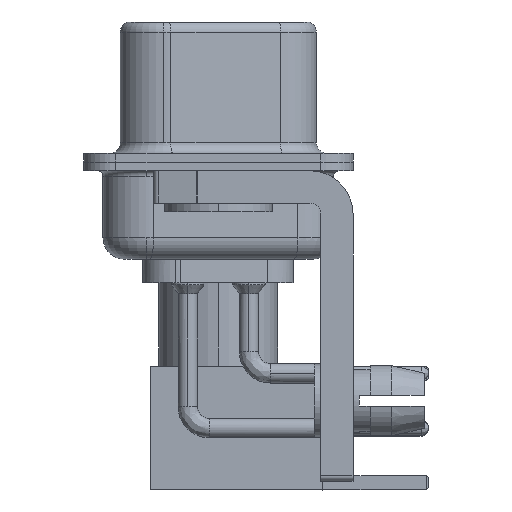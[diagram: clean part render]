
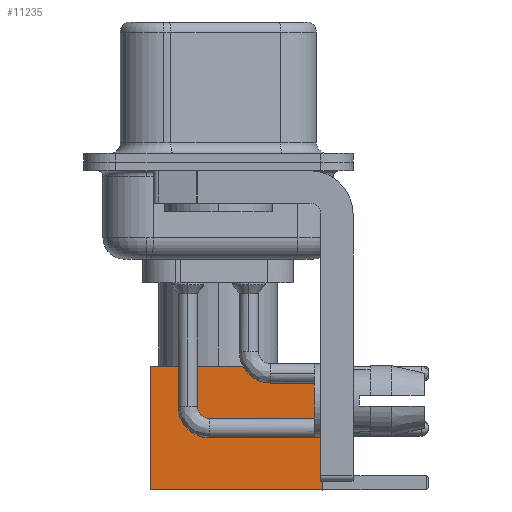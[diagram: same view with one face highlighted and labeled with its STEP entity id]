
A CAD part, left-side view. The second image highlights one B-rep face of the part: STEP entity #11235.
In plain terms, the highlighted face is planar.
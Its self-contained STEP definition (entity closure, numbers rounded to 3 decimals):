
#1261 = VERTEX_POINT ( 'NONE', #21179 ) ;
#3146 = VECTOR ( 'NONE', #19680, 1000. ) ;
#3464 = CARTESIAN_POINT ( 'NONE',  ( 2.875, 2.875, 0. ) ) ;
#3887 = DIRECTION ( 'NONE',  ( 0., 0., -1. ) ) ;
#3972 = VECTOR ( 'NONE', #4220, 1000. ) ;
#4220 = DIRECTION ( 'NONE',  ( 0., 0., -1. ) ) ;
#5386 = ORIENTED_EDGE ( 'NONE', *, *, #24501, .T. ) ;
#5910 = FACE_OUTER_BOUND ( 'NONE', #11796, .T. ) ;
#6385 = CARTESIAN_POINT ( 'NONE',  ( 2.875, 2.875, 8. ) ) ;
#6517 = CARTESIAN_POINT ( 'NONE',  ( 0., 2.875, 8. ) ) ;
#7740 = VERTEX_POINT ( 'NONE', #16381 ) ;
#8917 = LINE ( 'NONE', #17222, #3146 ) ;
#9050 = VERTEX_POINT ( 'NONE', #6385 ) ;
#9593 = VECTOR ( 'NONE', #17428, 1000. ) ;
#11180 = CARTESIAN_POINT ( 'NONE',  ( -2.875, 2.875, 0. ) ) ;
#11235 = ADVANCED_FACE ( 'NONE', ( #5910 ), #12590, .T. ) ;
#11389 = CARTESIAN_POINT ( 'NONE',  ( 2.875, 2.875, 0. ) ) ;
#11796 = EDGE_LOOP ( 'NONE', ( #25147, #5386, #18564, #21313 ) ) ;
#12316 = DIRECTION ( 'NONE',  ( 0., 1., 0. ) ) ;
#12590 = PLANE ( 'NONE',  #17521 ) ;
#13275 = VERTEX_POINT ( 'NONE', #11389 ) ;
#13364 = LINE ( 'NONE', #11180, #3972 ) ;
#14358 = DIRECTION ( 'NONE',  ( 0., 0., 1. ) ) ;
#14367 = CARTESIAN_POINT ( 'NONE',  ( 2.875, 2.875, 0. ) ) ;
#16381 = CARTESIAN_POINT ( 'NONE',  ( -2.875, 2.875, 0. ) ) ;
#17222 = CARTESIAN_POINT ( 'NONE',  ( 0., 2.875, 0. ) ) ;
#17428 = DIRECTION ( 'NONE',  ( -1., 0., 0. ) ) ;
#17521 = AXIS2_PLACEMENT_3D ( 'NONE', #3464, #12316, #14358 ) ;
#18148 = EDGE_CURVE ( 'NONE', #1261, #7740, #13364, .T. ) ;
#18564 = ORIENTED_EDGE ( 'NONE', *, *, #18148, .F. ) ;
#19680 = DIRECTION ( 'NONE',  ( -1., 0., 0. ) ) ;
#21179 = CARTESIAN_POINT ( 'NONE',  ( -2.875, 2.875, 8. ) ) ;
#21313 = ORIENTED_EDGE ( 'NONE', *, *, #23566, .F. ) ;
#22676 = VECTOR ( 'NONE', #3887, 1000. ) ;
#23518 = LINE ( 'NONE', #14367, #22676 ) ;
#23566 = EDGE_CURVE ( 'NONE', #9050, #1261, #28468, .T. ) ;
#24501 = EDGE_CURVE ( 'NONE', #13275, #7740, #8917, .T. ) ;
#25147 = ORIENTED_EDGE ( 'NONE', *, *, #26723, .T. ) ;
#26723 = EDGE_CURVE ( 'NONE', #9050, #13275, #23518, .T. ) ;
#28468 = LINE ( 'NONE', #6517, #9593 ) ;
